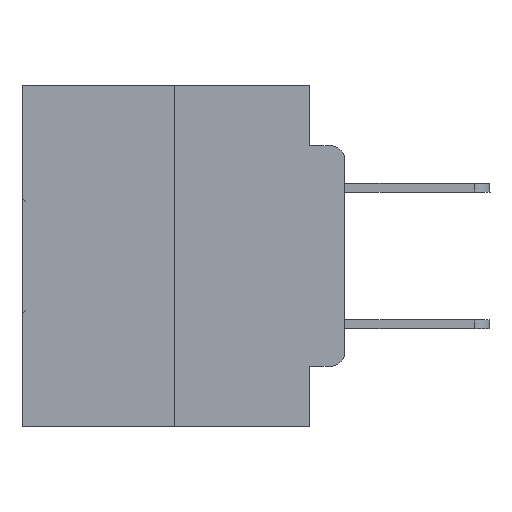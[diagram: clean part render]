
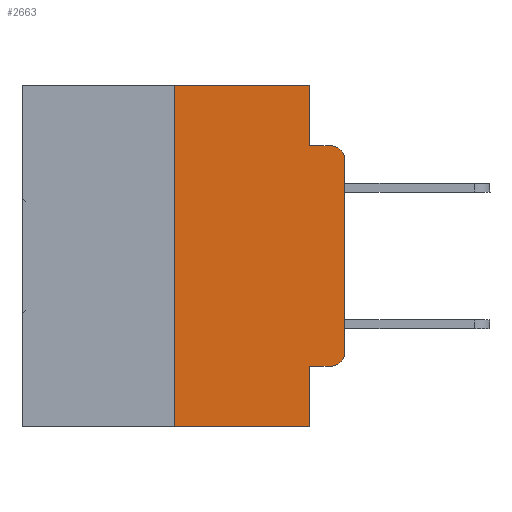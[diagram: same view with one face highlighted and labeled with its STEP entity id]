
A CAD part, left-side view. The second image highlights one B-rep face of the part: STEP entity #2663.
In plain terms, the highlighted planar face has unit normal (-1, 0, 0).
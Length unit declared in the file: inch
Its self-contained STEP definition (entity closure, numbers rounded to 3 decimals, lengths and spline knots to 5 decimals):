
#315 = CARTESIAN_POINT ( 'NONE',  ( 0., 0.051, -0.0885 ) ) ;
#557 = CIRCLE ( 'NONE', #23046, 0.02 ) ;
#577 = VERTEX_POINT ( 'NONE', #2656 ) ;
#979 = CARTESIAN_POINT ( 'NONE',  ( 0., 0.02, -0.4115 ) ) ;
#1476 = VERTEX_POINT ( 'NONE', #5574 ) ;
#1804 = DIRECTION ( 'NONE',  ( 0., 0., 1. ) ) ;
#1964 = CARTESIAN_POINT ( 'NONE',  ( 0., 0., 0. ) ) ;
#2028 = CARTESIAN_POINT ( 'NONE',  ( 0., 0.051, -0.4115 ) ) ;
#2330 = ORIENTED_EDGE ( 'NONE', *, *, #23328, .F. ) ;
#2404 = VERTEX_POINT ( 'NONE', #979 ) ;
#2487 = VERTEX_POINT ( 'NONE', #7072 ) ;
#2656 = CARTESIAN_POINT ( 'NONE',  ( 0., 0.02, -0.0885 ) ) ;
#2663 = ADVANCED_FACE ( 'NONE', ( #27348 ), #5144, .F. ) ;
#2895 = CARTESIAN_POINT ( 'NONE',  ( 0., 0.473, 0. ) ) ;
#3219 = DIRECTION ( 'NONE',  ( 0., 0., -1. ) ) ;
#3245 = VECTOR ( 'NONE', #28729, 39.37008 ) ;
#3289 = VECTOR ( 'NONE', #17908, 39.37008 ) ;
#3440 = LINE ( 'NONE', #16089, #11354 ) ;
#4217 = LINE ( 'NONE', #1964, #20311 ) ;
#4733 = EDGE_CURVE ( 'NONE', #2404, #2487, #13677, .T. ) ;
#5025 = VERTEX_POINT ( 'NONE', #8627 ) ;
#5144 = PLANE ( 'NONE',  #9491 ) ;
#5574 = CARTESIAN_POINT ( 'NONE',  ( 0., 0.25, 0. ) ) ;
#5620 = DIRECTION ( 'NONE',  ( -1., 0., 0. ) ) ;
#7070 = VECTOR ( 'NONE', #21632, 39.37008 ) ;
#7072 = CARTESIAN_POINT ( 'NONE',  ( 0., 0., -0.3915 ) ) ;
#7386 = CARTESIAN_POINT ( 'NONE',  ( 0., 0.473, 0. ) ) ;
#7703 = DIRECTION ( 'NONE',  ( 1., 0., 0. ) ) ;
#8079 = AXIS2_PLACEMENT_3D ( 'NONE', #31521, #27034, #16667 ) ;
#8627 = CARTESIAN_POINT ( 'NONE',  ( 0., 0., -0.1085 ) ) ;
#8788 = EDGE_CURVE ( 'NONE', #17881, #29234, #15355, .T. ) ;
#9246 = CARTESIAN_POINT ( 'NONE',  ( 0., 0.051, -0.0885 ) ) ;
#9491 = AXIS2_PLACEMENT_3D ( 'NONE', #2895, #7703, #3219 ) ;
#10223 = DIRECTION ( 'NONE',  ( 0., -1., 0. ) ) ;
#10227 = CARTESIAN_POINT ( 'NONE',  ( 0., 0.051, 0. ) ) ;
#11354 = VECTOR ( 'NONE', #20735, 39.37008 ) ;
#11390 = LINE ( 'NONE', #16828, #7070 ) ;
#12458 = ORIENTED_EDGE ( 'NONE', *, *, #15219, .F. ) ;
#12789 = LINE ( 'NONE', #27471, #27271 ) ;
#12834 = LINE ( 'NONE', #315, #24765 ) ;
#13544 = EDGE_CURVE ( 'NONE', #2487, #5025, #4217, .T. ) ;
#13677 = CIRCLE ( 'NONE', #8079, 0.02 ) ;
#14431 = CARTESIAN_POINT ( 'NONE',  ( 0., 0.25, -0.5 ) ) ;
#15219 = EDGE_CURVE ( 'NONE', #17160, #30314, #11390, .T. ) ;
#15286 = EDGE_LOOP ( 'NONE', ( #30569, #29423, #17597, #21805, #2330, #31003, #31058, #12458, #16105, #16142 ) ) ;
#15355 = LINE ( 'NONE', #10227, #3289 ) ;
#15386 = DIRECTION ( 'NONE',  ( 0., 0., -1. ) ) ;
#16089 = CARTESIAN_POINT ( 'NONE',  ( 0., 0.25, 0. ) ) ;
#16105 = ORIENTED_EDGE ( 'NONE', *, *, #29337, .T. ) ;
#16142 = ORIENTED_EDGE ( 'NONE', *, *, #4733, .T. ) ;
#16667 = DIRECTION ( 'NONE',  ( 0., 0., -1. ) ) ;
#16828 = CARTESIAN_POINT ( 'NONE',  ( 0., 0.051, 0. ) ) ;
#17160 = VERTEX_POINT ( 'NONE', #23530 ) ;
#17597 = ORIENTED_EDGE ( 'NONE', *, *, #29877, .F. ) ;
#17881 = VERTEX_POINT ( 'NONE', #19488 ) ;
#17908 = DIRECTION ( 'NONE',  ( 0., 0., -1. ) ) ;
#18701 = VERTEX_POINT ( 'NONE', #14431 ) ;
#19488 = CARTESIAN_POINT ( 'NONE',  ( 0., 0.051, 0. ) ) ;
#19888 = VECTOR ( 'NONE', #27188, 39.37008 ) ;
#20188 = LINE ( 'NONE', #7386, #19888 ) ;
#20198 = DIRECTION ( 'NONE',  ( 0., -1., 0. ) ) ;
#20311 = VECTOR ( 'NONE', #1804, 39.37008 ) ;
#20735 = DIRECTION ( 'NONE',  ( 0., 0., 1. ) ) ;
#21632 = DIRECTION ( 'NONE',  ( 0., 0., -1. ) ) ;
#21805 = ORIENTED_EDGE ( 'NONE', *, *, #8788, .F. ) ;
#22425 = CARTESIAN_POINT ( 'NONE',  ( 0., 0.02, -0.1085 ) ) ;
#23046 = AXIS2_PLACEMENT_3D ( 'NONE', #22425, #5620, #15386 ) ;
#23328 = EDGE_CURVE ( 'NONE', #1476, #17881, #20188, .T. ) ;
#23530 = CARTESIAN_POINT ( 'NONE',  ( 0., 0.051, -0.4115 ) ) ;
#24765 = VECTOR ( 'NONE', #20198, 39.37008 ) ;
#26799 = EDGE_CURVE ( 'NONE', #5025, #577, #557, .T. ) ;
#27034 = DIRECTION ( 'NONE',  ( -1., 0., 0. ) ) ;
#27188 = DIRECTION ( 'NONE',  ( 0., -1., 0. ) ) ;
#27271 = VECTOR ( 'NONE', #10223, 39.37008 ) ;
#27348 = FACE_OUTER_BOUND ( 'NONE', #15286, .T. ) ;
#27471 = CARTESIAN_POINT ( 'NONE',  ( 0., 0.473, -0.5 ) ) ;
#27896 = EDGE_CURVE ( 'NONE', #18701, #1476, #3440, .T. ) ;
#28245 = LINE ( 'NONE', #2028, #3245 ) ;
#28729 = DIRECTION ( 'NONE',  ( 0., -1., 0. ) ) ;
#29234 = VERTEX_POINT ( 'NONE', #9246 ) ;
#29337 = EDGE_CURVE ( 'NONE', #17160, #2404, #28245, .T. ) ;
#29423 = ORIENTED_EDGE ( 'NONE', *, *, #26799, .T. ) ;
#29732 = CARTESIAN_POINT ( 'NONE',  ( 0., 0.051, -0.5 ) ) ;
#29877 = EDGE_CURVE ( 'NONE', #29234, #577, #12834, .T. ) ;
#30300 = EDGE_CURVE ( 'NONE', #18701, #30314, #12789, .T. ) ;
#30314 = VERTEX_POINT ( 'NONE', #29732 ) ;
#30569 = ORIENTED_EDGE ( 'NONE', *, *, #13544, .T. ) ;
#31003 = ORIENTED_EDGE ( 'NONE', *, *, #27896, .F. ) ;
#31058 = ORIENTED_EDGE ( 'NONE', *, *, #30300, .T. ) ;
#31521 = CARTESIAN_POINT ( 'NONE',  ( 0., 0.02, -0.3915 ) ) ;
